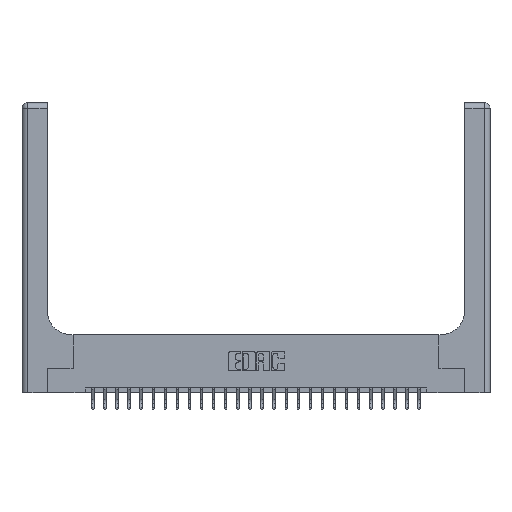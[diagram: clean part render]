
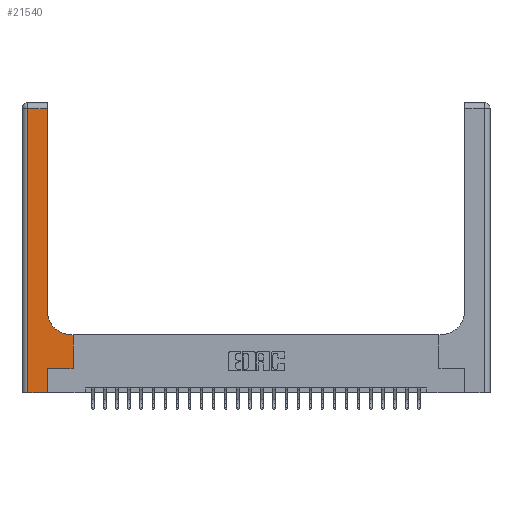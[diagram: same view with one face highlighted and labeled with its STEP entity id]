
A CAD part, top view. The second image highlights one B-rep face of the part: STEP entity #21540.
In plain terms, the highlighted planar face has unit normal (0, 0, 1).
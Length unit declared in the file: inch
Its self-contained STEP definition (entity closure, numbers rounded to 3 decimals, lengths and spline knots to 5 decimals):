
#163 = CARTESIAN_POINT ( 'NONE',  ( 0.06, 0., 0.37 ) ) ;
#1521 = CARTESIAN_POINT ( 'NONE',  ( 0.26, 2.94, 0.37 ) ) ;
#1767 = CARTESIAN_POINT ( 'NONE',  ( 0.265, 0., 0.37 ) ) ;
#1987 = CARTESIAN_POINT ( 'NONE',  ( 0.26, 0.6, 0.37 ) ) ;
#2036 = LINE ( 'NONE', #23608, #7907 ) ;
#2093 = VERTEX_POINT ( 'NONE', #4631 ) ;
#2281 = DIRECTION ( 'NONE',  ( -1., 0., 0. ) ) ;
#2711 = PLANE ( 'NONE',  #17809 ) ;
#3417 = VERTEX_POINT ( 'NONE', #1521 ) ;
#3943 = CARTESIAN_POINT ( 'NONE',  ( 0.51, 0.85, 0.37 ) ) ;
#4495 = CARTESIAN_POINT ( 'NONE',  ( 0.265, 0.25, 0.37 ) ) ;
#4631 = CARTESIAN_POINT ( 'NONE',  ( 0.26, 0.85, 0.37 ) ) ;
#4827 = DIRECTION ( 'NONE',  ( 0., 1., 0. ) ) ;
#5488 = EDGE_CURVE ( 'NONE', #25123, #19077, #24449, .T. ) ;
#6134 = VERTEX_POINT ( 'NONE', #25379 ) ;
#6232 = CARTESIAN_POINT ( 'NONE',  ( 0.06, 2.94, 0.37 ) ) ;
#6247 = LINE ( 'NONE', #16829, #8725 ) ;
#6713 = CARTESIAN_POINT ( 'NONE',  ( 0.528, 0.6, 0.37 ) ) ;
#7647 = ORIENTED_EDGE ( 'NONE', *, *, #13513, .T. ) ;
#7694 = EDGE_CURVE ( 'NONE', #14897, #2093, #16286, .T. ) ;
#7907 = VECTOR ( 'NONE', #21362, 39.37008 ) ;
#8108 = EDGE_CURVE ( 'NONE', #3417, #13049, #25244, .T. ) ;
#8725 = VECTOR ( 'NONE', #10760, 39.37008 ) ;
#8868 = VECTOR ( 'NONE', #2281, 39.37008 ) ;
#9100 = EDGE_CURVE ( 'NONE', #6134, #25123, #19949, .T. ) ;
#9545 = ORIENTED_EDGE ( 'NONE', *, *, #22681, .T. ) ;
#9753 = DIRECTION ( 'NONE',  ( 0., 1., 0. ) ) ;
#9771 = LINE ( 'NONE', #16624, #19070 ) ;
#10331 = CARTESIAN_POINT ( 'NONE',  ( 0.265, 0.25, 0.37 ) ) ;
#10760 = DIRECTION ( 'NONE',  ( 0., 1., 0. ) ) ;
#11334 = VECTOR ( 'NONE', #19487, 39.37008 ) ;
#11479 = EDGE_CURVE ( 'NONE', #19077, #22322, #6247, .T. ) ;
#12009 = DIRECTION ( 'NONE',  ( 1., 0., 0. ) ) ;
#12613 = FACE_OUTER_BOUND ( 'NONE', #15314, .T. ) ;
#13049 = VERTEX_POINT ( 'NONE', #6232 ) ;
#13275 = VECTOR ( 'NONE', #21415, 39.37008 ) ;
#13513 = EDGE_CURVE ( 'NONE', #22322, #14897, #15158, .T. ) ;
#13563 = VERTEX_POINT ( 'NONE', #163 ) ;
#13766 = DIRECTION ( 'NONE',  ( 0., 0., -1. ) ) ;
#13944 = CARTESIAN_POINT ( 'NONE',  ( 0., 0., 0.37 ) ) ;
#14327 = DIRECTION ( 'NONE',  ( -1., 0., 0. ) ) ;
#14405 = ORIENTED_EDGE ( 'NONE', *, *, #16773, .T. ) ;
#14586 = ORIENTED_EDGE ( 'NONE', *, *, #5488, .T. ) ;
#14897 = VERTEX_POINT ( 'NONE', #18231 ) ;
#15158 = LINE ( 'NONE', #1987, #13275 ) ;
#15237 = ORIENTED_EDGE ( 'NONE', *, *, #9100, .T. ) ;
#15314 = EDGE_LOOP ( 'NONE', ( #25100, #25370, #14405, #9545, #15237, #14586, #23169, #7647, #23300 ) ) ;
#15840 = EDGE_CURVE ( 'NONE', #2093, #3417, #9771, .T. ) ;
#16082 = VECTOR ( 'NONE', #20540, 39.37008 ) ;
#16286 = CIRCLE ( 'NONE', #23911, 0.25 ) ;
#16614 = LINE ( 'NONE', #13944, #11334 ) ;
#16624 = CARTESIAN_POINT ( 'NONE',  ( 0.26, 3., 0.37 ) ) ;
#16773 = EDGE_CURVE ( 'NONE', #13049, #13563, #2036, .T. ) ;
#16829 = CARTESIAN_POINT ( 'NONE',  ( 0.528, 0.25, 0.37 ) ) ;
#17809 = AXIS2_PLACEMENT_3D ( 'NONE', #24380, #18494, #14327 ) ;
#18231 = CARTESIAN_POINT ( 'NONE',  ( 0.51, 0.6, 0.37 ) ) ;
#18494 = DIRECTION ( 'NONE',  ( 0., 0., -1. ) ) ;
#19070 = VECTOR ( 'NONE', #4827, 39.37008 ) ;
#19077 = VERTEX_POINT ( 'NONE', #22773 ) ;
#19487 = DIRECTION ( 'NONE',  ( 1., 0., 0. ) ) ;
#19949 = LINE ( 'NONE', #1767, #21481 ) ;
#20540 = DIRECTION ( 'NONE',  ( 1., 0., 0. ) ) ;
#21362 = DIRECTION ( 'NONE',  ( 0., -1., 0. ) ) ;
#21415 = DIRECTION ( 'NONE',  ( -1., 0., 0. ) ) ;
#21481 = VECTOR ( 'NONE', #9753, 39.37008 ) ;
#21540 = ADVANCED_FACE ( 'NONE', ( #12613 ), #2711, .F. ) ;
#22322 = VERTEX_POINT ( 'NONE', #6713 ) ;
#22681 = EDGE_CURVE ( 'NONE', #13563, #6134, #16614, .T. ) ;
#22773 = CARTESIAN_POINT ( 'NONE',  ( 0.528, 0.25, 0.37 ) ) ;
#23169 = ORIENTED_EDGE ( 'NONE', *, *, #11479, .T. ) ;
#23300 = ORIENTED_EDGE ( 'NONE', *, *, #7694, .T. ) ;
#23608 = CARTESIAN_POINT ( 'NONE',  ( 0.06, 3., 0.37 ) ) ;
#23911 = AXIS2_PLACEMENT_3D ( 'NONE', #3943, #13766, #12009 ) ;
#24380 = CARTESIAN_POINT ( 'NONE',  ( 0., 3., 0.37 ) ) ;
#24449 = LINE ( 'NONE', #4495, #16082 ) ;
#25100 = ORIENTED_EDGE ( 'NONE', *, *, #15840, .T. ) ;
#25123 = VERTEX_POINT ( 'NONE', #10331 ) ;
#25244 = LINE ( 'NONE', #25321, #8868 ) ;
#25321 = CARTESIAN_POINT ( 'NONE',  ( 0., 2.94, 0.37 ) ) ;
#25370 = ORIENTED_EDGE ( 'NONE', *, *, #8108, .T. ) ;
#25379 = CARTESIAN_POINT ( 'NONE',  ( 0.265, 0., 0.37 ) ) ;
